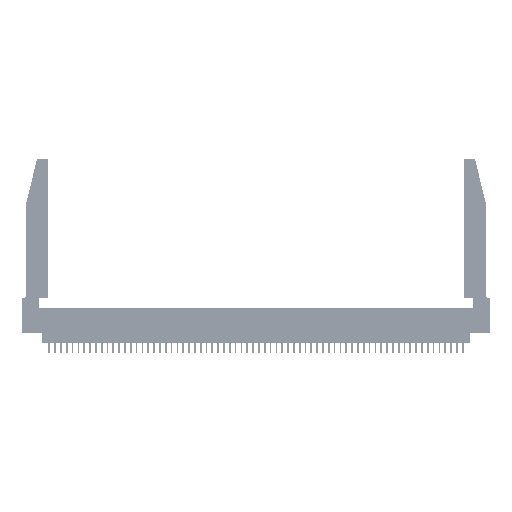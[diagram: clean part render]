
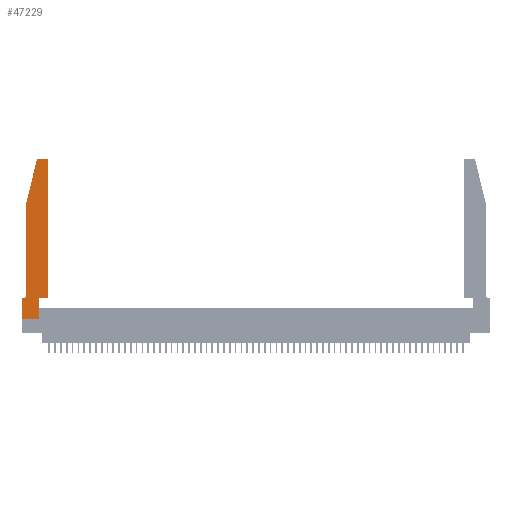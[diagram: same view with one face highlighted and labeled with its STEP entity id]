
A CAD part, top view. The second image highlights one B-rep face of the part: STEP entity #47229.
In plain terms, the highlighted planar face has unit normal (0, 0, 1).
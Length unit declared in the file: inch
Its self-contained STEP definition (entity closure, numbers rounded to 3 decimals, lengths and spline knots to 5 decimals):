
#91 = VERTEX_POINT ( 'NONE', #48856 ) ;
#767 = EDGE_CURVE ( 'NONE', #47863, #34875, #7394, .T. ) ;
#1426 = CIRCLE ( 'NONE', #35502, 0.07 ) ;
#1680 = CIRCLE ( 'NONE', #7689, 0.03 ) ;
#1780 = LINE ( 'NONE', #39675, #49050 ) ;
#4125 = LINE ( 'NONE', #28829, #31934 ) ;
#4591 = VERTEX_POINT ( 'NONE', #14137 ) ;
#4875 = CARTESIAN_POINT ( 'NONE',  ( 0.2605, 2.75, 0.37 ) ) ;
#5017 = CARTESIAN_POINT ( 'NONE',  ( 0., 0.35, 0.37 ) ) ;
#5037 = CARTESIAN_POINT ( 'NONE',  ( 0., 0.35, 0.37 ) ) ;
#5543 = CARTESIAN_POINT ( 'NONE',  ( 0.0755, 2., 0.37 ) ) ;
#5592 = CARTESIAN_POINT ( 'NONE',  ( 0.0755, 0.42, 0.37 ) ) ;
#6020 = ORIENTED_EDGE ( 'NONE', *, *, #47789, .T. ) ;
#6217 = DIRECTION ( 'NONE',  ( 0., 0., 1. ) ) ;
#6353 = CARTESIAN_POINT ( 'NONE',  ( 0.0755, 0.35, 0.37 ) ) ;
#6620 = CARTESIAN_POINT ( 'NONE',  ( 0.4205, 2.72, 0.37 ) ) ;
#6712 = VECTOR ( 'NONE', #54212, 39.37008 ) ;
#6795 = CARTESIAN_POINT ( 'NONE',  ( 0.284, 2.75, 0.37 ) ) ;
#7394 = LINE ( 'NONE', #4875, #6712 ) ;
#7491 = DIRECTION ( 'NONE',  ( 0., 0., 1. ) ) ;
#7689 = AXIS2_PLACEMENT_3D ( 'NONE', #6620, #6217, #37642 ) ;
#9567 = ORIENTED_EDGE ( 'NONE', *, *, #31210, .T. ) ;
#9855 = FACE_OUTER_BOUND ( 'NONE', #56320, .T. ) ;
#10879 = AXIS2_PLACEMENT_3D ( 'NONE', #11370, #7491, #43228 ) ;
#11370 = CARTESIAN_POINT ( 'NONE',  ( 0.284, 2.72, 0.37 ) ) ;
#12868 = VERTEX_POINT ( 'NONE', #30105 ) ;
#12956 = DIRECTION ( 'NONE',  ( -1., 0., 0. ) ) ;
#14030 = EDGE_CURVE ( 'NONE', #34875, #12868, #16024, .T. ) ;
#14137 = CARTESIAN_POINT ( 'NONE',  ( 0.4505, 0.35, 0.37 ) ) ;
#14835 = DIRECTION ( 'NONE',  ( 1., 0., 0. ) ) ;
#16024 = CIRCLE ( 'NONE', #10879, 0.03 ) ;
#16107 = AXIS2_PLACEMENT_3D ( 'NONE', #5017, #26965, #32166 ) ;
#16576 = VECTOR ( 'NONE', #32921, 39.37008 ) ;
#17240 = CARTESIAN_POINT ( 'NONE',  ( 0.0055, 0.42, 0.37 ) ) ;
#18206 = CARTESIAN_POINT ( 'NONE',  ( 0.4505, 0.35, 0.37 ) ) ;
#19924 = ORIENTED_EDGE ( 'NONE', *, *, #767, .T. ) ;
#20360 = LINE ( 'NONE', #25106, #27229 ) ;
#20566 = CARTESIAN_POINT ( 'NONE',  ( 0.4505, 2.72, 0.37 ) ) ;
#21209 = LINE ( 'NONE', #18206, #42074 ) ;
#21443 = VERTEX_POINT ( 'NONE', #20566 ) ;
#21646 = EDGE_CURVE ( 'NONE', #51648, #4591, #21209, .T. ) ;
#21873 = DIRECTION ( 'NONE',  ( 0., -1., 0. ) ) ;
#22996 = EDGE_CURVE ( 'NONE', #28405, #51648, #24010, .T. ) ;
#24010 = LINE ( 'NONE', #48163, #51023 ) ;
#24408 = LINE ( 'NONE', #5543, #35431 ) ;
#24522 = ORIENTED_EDGE ( 'NONE', *, *, #27183, .T. ) ;
#25106 = CARTESIAN_POINT ( 'NONE',  ( 0.4505, 0.35, 0.37 ) ) ;
#26306 = EDGE_CURVE ( 'NONE', #21443, #47863, #1680, .T. ) ;
#26333 = ORIENTED_EDGE ( 'NONE', *, *, #33331, .T. ) ;
#26965 = DIRECTION ( 'NONE',  ( 0., 0., 1. ) ) ;
#27183 = EDGE_CURVE ( 'NONE', #4591, #21443, #20360, .T. ) ;
#27229 = VECTOR ( 'NONE', #46685, 39.37008 ) ;
#28405 = VERTEX_POINT ( 'NONE', #28643 ) ;
#28643 = CARTESIAN_POINT ( 'NONE',  ( 0.2865, 0., 0.37 ) ) ;
#28723 = ORIENTED_EDGE ( 'NONE', *, *, #22996, .T. ) ;
#28829 = CARTESIAN_POINT ( 'NONE',  ( 0.0755, 2., 0.37 ) ) ;
#28912 = ORIENTED_EDGE ( 'NONE', *, *, #14030, .T. ) ;
#30105 = CARTESIAN_POINT ( 'NONE',  ( 0.25487, 2.72718, 0.37 ) ) ;
#30332 = ORIENTED_EDGE ( 'NONE', *, *, #37509, .T. ) ;
#31210 = EDGE_CURVE ( 'NONE', #91, #28405, #35433, .T. ) ;
#31598 = PLANE ( 'NONE',  #16107 ) ;
#31934 = VECTOR ( 'NONE', #41888, 39.37008 ) ;
#32166 = DIRECTION ( 'NONE',  ( 1., 0., 0. ) ) ;
#32617 = CARTESIAN_POINT ( 'NONE',  ( 0., 0., 0.37 ) ) ;
#32921 = DIRECTION ( 'NONE',  ( -1., 0., 0. ) ) ;
#33331 = EDGE_CURVE ( 'NONE', #49259, #36256, #52001, .T. ) ;
#34819 = ORIENTED_EDGE ( 'NONE', *, *, #26306, .T. ) ;
#34875 = VERTEX_POINT ( 'NONE', #6795 ) ;
#35431 = VECTOR ( 'NONE', #21873, 39.37008 ) ;
#35433 = LINE ( 'NONE', #32617, #43867 ) ;
#35502 = AXIS2_PLACEMENT_3D ( 'NONE', #17240, #57404, #12956 ) ;
#36256 = VERTEX_POINT ( 'NONE', #5037 ) ;
#37509 = EDGE_CURVE ( 'NONE', #36256, #91, #1780, .T. ) ;
#37642 = DIRECTION ( 'NONE',  ( 1., 0., 0. ) ) ;
#37683 = CARTESIAN_POINT ( 'NONE',  ( 0.0055, 0.35, 0.37 ) ) ;
#37931 = ORIENTED_EDGE ( 'NONE', *, *, #47953, .T. ) ;
#39083 = ORIENTED_EDGE ( 'NONE', *, *, #52555, .T. ) ;
#39394 = DIRECTION ( 'NONE',  ( 0., 1., 0. ) ) ;
#39675 = CARTESIAN_POINT ( 'NONE',  ( 0., 0., 0.37 ) ) ;
#41262 = VERTEX_POINT ( 'NONE', #52059 ) ;
#41888 = DIRECTION ( 'NONE',  ( -0.239, -0.971, 0. ) ) ;
#42074 = VECTOR ( 'NONE', #52753, 39.37008 ) ;
#42407 = CARTESIAN_POINT ( 'NONE',  ( 0.2865, 0.35, 0.37 ) ) ;
#43228 = DIRECTION ( 'NONE',  ( 1., 0., 0. ) ) ;
#43867 = VECTOR ( 'NONE', #14835, 39.37008 ) ;
#46229 = ORIENTED_EDGE ( 'NONE', *, *, #21646, .T. ) ;
#46685 = DIRECTION ( 'NONE',  ( 0., 1., 0. ) ) ;
#47229 = ADVANCED_FACE ( 'NONE', ( #9855 ), #31598, .T. ) ;
#47789 = EDGE_CURVE ( 'NONE', #41262, #54041, #24408, .T. ) ;
#47863 = VERTEX_POINT ( 'NONE', #53332 ) ;
#47953 = EDGE_CURVE ( 'NONE', #12868, #41262, #4125, .T. ) ;
#48163 = CARTESIAN_POINT ( 'NONE',  ( 0.2865, 0.35, 0.37 ) ) ;
#48856 = CARTESIAN_POINT ( 'NONE',  ( 0., 0., 0.37 ) ) ;
#49050 = VECTOR ( 'NONE', #52893, 39.37008 ) ;
#49259 = VERTEX_POINT ( 'NONE', #37683 ) ;
#51023 = VECTOR ( 'NONE', #39394, 39.37008 ) ;
#51648 = VERTEX_POINT ( 'NONE', #42407 ) ;
#52001 = LINE ( 'NONE', #6353, #16576 ) ;
#52059 = CARTESIAN_POINT ( 'NONE',  ( 0.0755, 2., 0.37 ) ) ;
#52555 = EDGE_CURVE ( 'NONE', #54041, #49259, #1426, .T. ) ;
#52753 = DIRECTION ( 'NONE',  ( 1., 0., 0. ) ) ;
#52893 = DIRECTION ( 'NONE',  ( 0., -1., 0. ) ) ;
#53332 = CARTESIAN_POINT ( 'NONE',  ( 0.4205, 2.75, 0.37 ) ) ;
#54041 = VERTEX_POINT ( 'NONE', #5592 ) ;
#54212 = DIRECTION ( 'NONE',  ( -1., 0., 0. ) ) ;
#56320 = EDGE_LOOP ( 'NONE', ( #19924, #28912, #37931, #6020, #39083, #26333, #30332, #9567, #28723, #46229, #24522, #34819 ) ) ;
#57404 = DIRECTION ( 'NONE',  ( 0., 0., -1. ) ) ;
